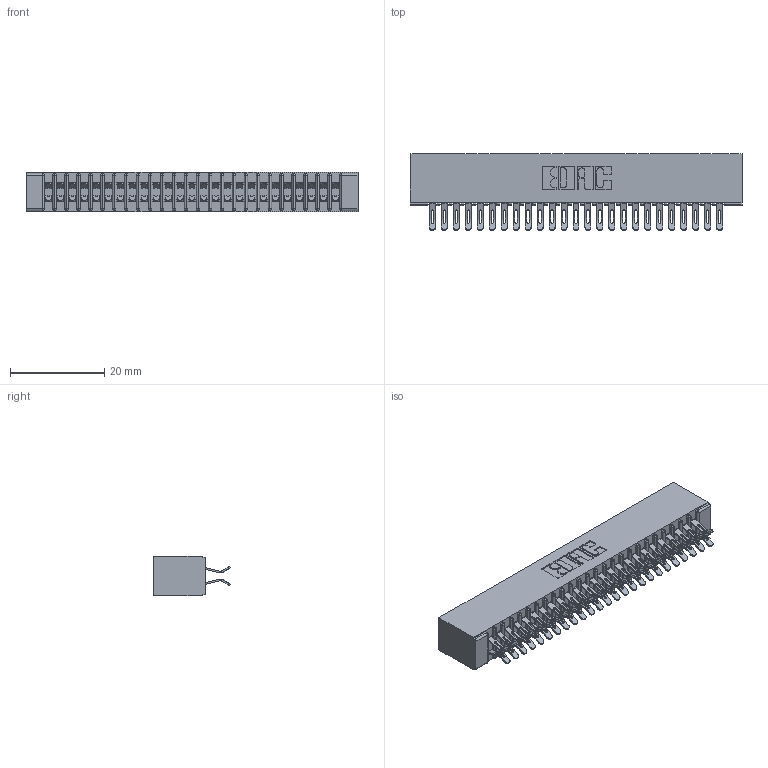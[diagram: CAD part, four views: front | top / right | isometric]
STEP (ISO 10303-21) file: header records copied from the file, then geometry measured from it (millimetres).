
FILE_DESCRIPTION (( 'STEP AP203' ), '1' );
FILE_NAME ('341-050-555-201.STEP', '2018-08-07T12:39:18', ( '' ), ( '' ), 'SwSTEP 2.0', 'SolidWorks 2016', '' );
FILE_SCHEMA (( 'CONFIG_CONTROL_DESIGN' ));
Length unit declared in the file: inch
Products named in the file (3): 341-050-555-201; 341 Part_No Mounting Lugs; 341-292-001_341-292-155
Assembly tree (51 placements, depth 2):
  341-050-555-201
    341 Part_No Mounting Lugs
    341-292-001_341-292-155  x50
Bounding box: 70.48 x 16.31 x 8.38 mm (x, y, z)
Volume: 4197 mm3; surface area: 9990.6 mm2
Topology: 51 solids, 51 shells, 4008 faces, 11967 edges, 7790 vertices
Faces by surface type: plane 2164, cylinder 1744, sphere 52, torus 48
Entity records: 32712 total; most frequent: CARTESIAN_POINT 5453, ORIENTED_EDGE 5406, DIRECTION 5293, EDGE_CURVE 2703, LINE 2153, VECTOR 2153, VERTEX_POINT 1714, AXIS2_PLACEMENT_3D 1570
